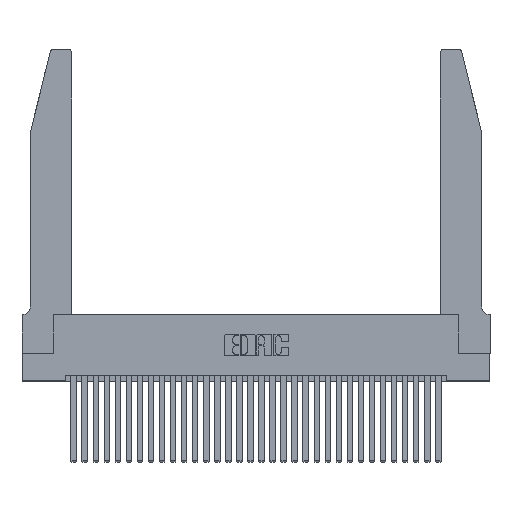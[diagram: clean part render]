
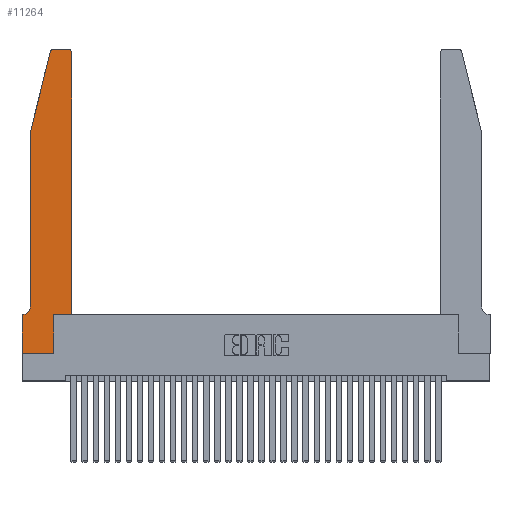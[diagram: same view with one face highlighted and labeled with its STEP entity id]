
A CAD part, top view. The second image highlights one B-rep face of the part: STEP entity #11264.
In plain terms, the highlighted planar face has unit normal (0, 0, 1).
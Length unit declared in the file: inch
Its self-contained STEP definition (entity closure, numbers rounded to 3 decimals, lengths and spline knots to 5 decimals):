
#55 = VECTOR ( 'NONE', #13702, 39.37008 ) ;
#857 = DIRECTION ( 'NONE',  ( 1., 0., 0. ) ) ;
#919 = EDGE_CURVE ( 'NONE', #10525, #8665, #17457, .T. ) ;
#1104 = EDGE_CURVE ( 'NONE', #21606, #27561, #17832, .T. ) ;
#1132 = CARTESIAN_POINT ( 'NONE',  ( 0.2865, 0., 0.37 ) ) ;
#1177 = CARTESIAN_POINT ( 'NONE',  ( 0.25487, 2.72718, 0.37 ) ) ;
#2790 = EDGE_CURVE ( 'NONE', #17227, #8514, #3216, .T. ) ;
#3028 = ORIENTED_EDGE ( 'NONE', *, *, #12117, .T. ) ;
#3216 = LINE ( 'NONE', #21433, #9108 ) ;
#3230 = EDGE_CURVE ( 'NONE', #29202, #7445, #6050, .T. ) ;
#4145 = CARTESIAN_POINT ( 'NONE',  ( 0.284, 2.75, 0.37 ) ) ;
#4546 = VERTEX_POINT ( 'NONE', #16461 ) ;
#4960 = DIRECTION ( 'NONE',  ( -1., 0., 0. ) ) ;
#5400 = CARTESIAN_POINT ( 'NONE',  ( 0., 0., 0.37 ) ) ;
#5401 = AXIS2_PLACEMENT_3D ( 'NONE', #12372, #14854, #32231 ) ;
#5842 = VECTOR ( 'NONE', #13421, 39.37008 ) ;
#5949 = DIRECTION ( 'NONE',  ( 0., 0., -1. ) ) ;
#5951 = DIRECTION ( 'NONE',  ( 1., 0., 0. ) ) ;
#6050 = LINE ( 'NONE', #26179, #24354 ) ;
#6241 = ORIENTED_EDGE ( 'NONE', *, *, #24570, .T. ) ;
#7212 = LINE ( 'NONE', #28542, #7992 ) ;
#7445 = VERTEX_POINT ( 'NONE', #27914 ) ;
#7906 = DIRECTION ( 'NONE',  ( 1., 0., 0. ) ) ;
#7992 = VECTOR ( 'NONE', #11165, 39.37008 ) ;
#8133 = CARTESIAN_POINT ( 'NONE',  ( 0.0755, 0.42, 0.37 ) ) ;
#8514 = VERTEX_POINT ( 'NONE', #8133 ) ;
#8665 = VERTEX_POINT ( 'NONE', #1177 ) ;
#9108 = VECTOR ( 'NONE', #23926, 39.37008 ) ;
#9157 = VERTEX_POINT ( 'NONE', #30713 ) ;
#10146 = EDGE_LOOP ( 'NONE', ( #19092, #14055, #27252, #22200, #3028, #16365, #11319, #17935, #6241, #12939, #14469, #27673 ) ) ;
#10525 = VERTEX_POINT ( 'NONE', #4145 ) ;
#10851 = VECTOR ( 'NONE', #7906, 39.37008 ) ;
#10913 = EDGE_CURVE ( 'NONE', #8665, #17227, #7212, .T. ) ;
#11165 = DIRECTION ( 'NONE',  ( -0.239, -0.971, 0. ) ) ;
#11172 = CARTESIAN_POINT ( 'NONE',  ( 0.0755, 0.35, 0.37 ) ) ;
#11264 = ADVANCED_FACE ( 'NONE', ( #22786 ), #19741, .T. ) ;
#11319 = ORIENTED_EDGE ( 'NONE', *, *, #1104, .T. ) ;
#11949 = VECTOR ( 'NONE', #4960, 39.37008 ) ;
#12117 = EDGE_CURVE ( 'NONE', #8514, #28090, #15720, .T. ) ;
#12340 = CARTESIAN_POINT ( 'NONE',  ( 0., 0., 0.37 ) ) ;
#12372 = CARTESIAN_POINT ( 'NONE',  ( 0., 0.35, 0.37 ) ) ;
#12939 = ORIENTED_EDGE ( 'NONE', *, *, #20218, .T. ) ;
#13421 = DIRECTION ( 'NONE',  ( 0., 1., 0. ) ) ;
#13556 = VECTOR ( 'NONE', #5951, 39.37008 ) ;
#13702 = DIRECTION ( 'NONE',  ( -1., 0., 0. ) ) ;
#14055 = ORIENTED_EDGE ( 'NONE', *, *, #919, .T. ) ;
#14145 = CARTESIAN_POINT ( 'NONE',  ( 0.0055, 0.35, 0.37 ) ) ;
#14469 = ORIENTED_EDGE ( 'NONE', *, *, #3230, .T. ) ;
#14854 = DIRECTION ( 'NONE',  ( 0., 0., 1. ) ) ;
#15720 = CIRCLE ( 'NONE', #27528, 0.07 ) ;
#15874 = CARTESIAN_POINT ( 'NONE',  ( 0.4505, 0.35, 0.37 ) ) ;
#15891 = DIRECTION ( 'NONE',  ( 0., 0., 1. ) ) ;
#16365 = ORIENTED_EDGE ( 'NONE', *, *, #21666, .T. ) ;
#16461 = CARTESIAN_POINT ( 'NONE',  ( 0.2865, 0.35, 0.37 ) ) ;
#17227 = VERTEX_POINT ( 'NONE', #26020 ) ;
#17396 = CARTESIAN_POINT ( 'NONE',  ( 0.2605, 2.75, 0.37 ) ) ;
#17457 = CIRCLE ( 'NONE', #21912, 0.03 ) ;
#17464 = LINE ( 'NONE', #5400, #10851 ) ;
#17719 = EDGE_CURVE ( 'NONE', #7445, #9157, #19280, .T. ) ;
#17832 = LINE ( 'NONE', #23495, #18605 ) ;
#17833 = DIRECTION ( 'NONE',  ( 0., -1., 0. ) ) ;
#17935 = ORIENTED_EDGE ( 'NONE', *, *, #31312, .T. ) ;
#18538 = LINE ( 'NONE', #17396, #11949 ) ;
#18605 = VECTOR ( 'NONE', #17833, 39.37008 ) ;
#19041 = VERTEX_POINT ( 'NONE', #1132 ) ;
#19092 = ORIENTED_EDGE ( 'NONE', *, *, #26261, .T. ) ;
#19280 = CIRCLE ( 'NONE', #23075, 0.03 ) ;
#19741 = PLANE ( 'NONE',  #5401 ) ;
#20035 = LINE ( 'NONE', #11172, #55 ) ;
#20218 = EDGE_CURVE ( 'NONE', #4546, #29202, #27513, .T. ) ;
#20894 = CARTESIAN_POINT ( 'NONE',  ( 0.0055, 0.42, 0.37 ) ) ;
#21433 = CARTESIAN_POINT ( 'NONE',  ( 0.0755, 2., 0.37 ) ) ;
#21606 = VERTEX_POINT ( 'NONE', #23343 ) ;
#21666 = EDGE_CURVE ( 'NONE', #28090, #21606, #20035, .T. ) ;
#21912 = AXIS2_PLACEMENT_3D ( 'NONE', #22434, #24182, #23819 ) ;
#22200 = ORIENTED_EDGE ( 'NONE', *, *, #2790, .T. ) ;
#22434 = CARTESIAN_POINT ( 'NONE',  ( 0.284, 2.72, 0.37 ) ) ;
#22786 = FACE_OUTER_BOUND ( 'NONE', #10146, .T. ) ;
#23075 = AXIS2_PLACEMENT_3D ( 'NONE', #30759, #15891, #857 ) ;
#23299 = CARTESIAN_POINT ( 'NONE',  ( 0.4505, 0.35, 0.37 ) ) ;
#23343 = CARTESIAN_POINT ( 'NONE',  ( 0., 0.35, 0.37 ) ) ;
#23368 = DIRECTION ( 'NONE',  ( -1., 0., 0. ) ) ;
#23495 = CARTESIAN_POINT ( 'NONE',  ( 0., 0., 0.37 ) ) ;
#23819 = DIRECTION ( 'NONE',  ( 1., 0., 0. ) ) ;
#23926 = DIRECTION ( 'NONE',  ( 0., -1., 0. ) ) ;
#24182 = DIRECTION ( 'NONE',  ( 0., 0., 1. ) ) ;
#24354 = VECTOR ( 'NONE', #28685, 39.37008 ) ;
#24570 = EDGE_CURVE ( 'NONE', #19041, #4546, #31535, .T. ) ;
#26020 = CARTESIAN_POINT ( 'NONE',  ( 0.0755, 2., 0.37 ) ) ;
#26179 = CARTESIAN_POINT ( 'NONE',  ( 0.4505, 0.35, 0.37 ) ) ;
#26261 = EDGE_CURVE ( 'NONE', #9157, #10525, #18538, .T. ) ;
#27252 = ORIENTED_EDGE ( 'NONE', *, *, #10913, .T. ) ;
#27513 = LINE ( 'NONE', #15874, #13556 ) ;
#27528 = AXIS2_PLACEMENT_3D ( 'NONE', #20894, #5949, #23368 ) ;
#27561 = VERTEX_POINT ( 'NONE', #12340 ) ;
#27673 = ORIENTED_EDGE ( 'NONE', *, *, #17719, .T. ) ;
#27914 = CARTESIAN_POINT ( 'NONE',  ( 0.4505, 2.72, 0.37 ) ) ;
#28090 = VERTEX_POINT ( 'NONE', #14145 ) ;
#28542 = CARTESIAN_POINT ( 'NONE',  ( 0.0755, 2., 0.37 ) ) ;
#28685 = DIRECTION ( 'NONE',  ( 0., 1., 0. ) ) ;
#29202 = VERTEX_POINT ( 'NONE', #23299 ) ;
#30713 = CARTESIAN_POINT ( 'NONE',  ( 0.4205, 2.75, 0.37 ) ) ;
#30739 = CARTESIAN_POINT ( 'NONE',  ( 0.2865, 0.35, 0.37 ) ) ;
#30759 = CARTESIAN_POINT ( 'NONE',  ( 0.4205, 2.72, 0.37 ) ) ;
#31312 = EDGE_CURVE ( 'NONE', #27561, #19041, #17464, .T. ) ;
#31535 = LINE ( 'NONE', #30739, #5842 ) ;
#32231 = DIRECTION ( 'NONE',  ( 1., 0., 0. ) ) ;
